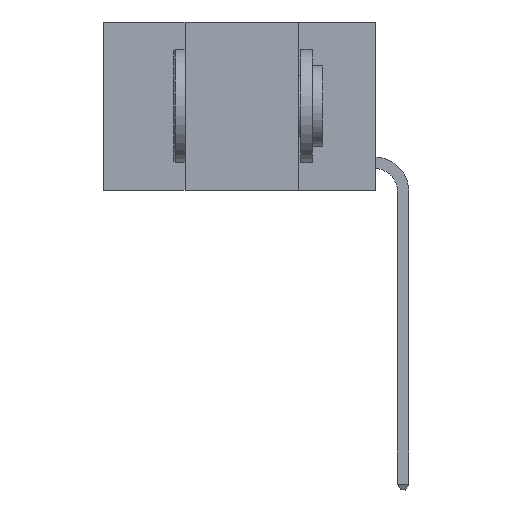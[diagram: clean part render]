
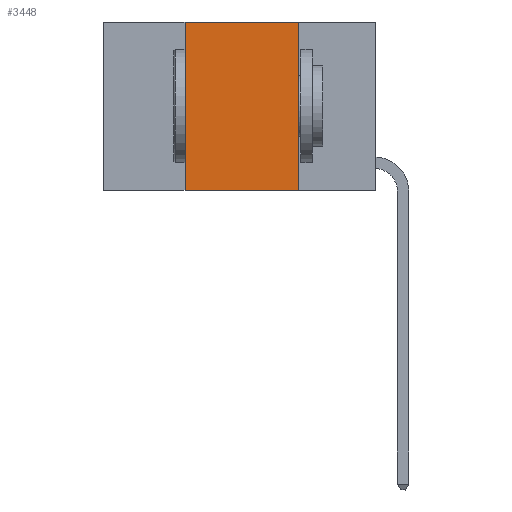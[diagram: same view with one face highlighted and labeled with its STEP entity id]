
A CAD part, left-side view. The second image highlights one B-rep face of the part: STEP entity #3448.
In plain terms, the highlighted planar face has unit normal (-1, 0, 0).
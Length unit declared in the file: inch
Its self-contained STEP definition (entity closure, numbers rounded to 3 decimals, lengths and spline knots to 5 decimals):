
#687 = EDGE_CURVE ( 'NONE', #4513, #5849, #4733, .T. ) ;
#817 = VECTOR ( 'NONE', #2018, 39.37008 ) ;
#1158 = VECTOR ( 'NONE', #10260, 39.37008 ) ;
#2018 = DIRECTION ( 'NONE',  ( 0., -1., 0. ) ) ;
#2038 = VERTEX_POINT ( 'NONE', #10872 ) ;
#2383 = ORIENTED_EDGE ( 'NONE', *, *, #13498, .F. ) ;
#2482 = ORIENTED_EDGE ( 'NONE', *, *, #4453, .F. ) ;
#3216 = PLANE ( 'NONE',  #8801 ) ;
#3448 = ADVANCED_FACE ( 'NONE', ( #8709 ), #3216, .F. ) ;
#3645 = ORIENTED_EDGE ( 'NONE', *, *, #687, .F. ) ;
#3662 = ORIENTED_EDGE ( 'NONE', *, *, #15948, .T. ) ;
#4453 = EDGE_CURVE ( 'NONE', #5849, #2038, #7474, .T. ) ;
#4513 = VERTEX_POINT ( 'NONE', #4835 ) ;
#4561 = DIRECTION ( 'NONE',  ( 1., 0., 0. ) ) ;
#4733 = LINE ( 'NONE', #6243, #1158 ) ;
#4770 = DIRECTION ( 'NONE',  ( 0., -1., 0. ) ) ;
#4835 = CARTESIAN_POINT ( 'NONE',  ( 0., 0.42, -0.37 ) ) ;
#4949 = VECTOR ( 'NONE', #4770, 39.37008 ) ;
#5364 = LINE ( 'NONE', #11214, #4949 ) ;
#5849 = VERTEX_POINT ( 'NONE', #7764 ) ;
#6049 = DIRECTION ( 'NONE',  ( 0., 0., -1. ) ) ;
#6243 = CARTESIAN_POINT ( 'NONE',  ( 0., 0.42, 0. ) ) ;
#6273 = LINE ( 'NONE', #11174, #12700 ) ;
#7474 = LINE ( 'NONE', #14957, #817 ) ;
#7544 = CARTESIAN_POINT ( 'NONE',  ( 0., 0.17, -0.37 ) ) ;
#7764 = CARTESIAN_POINT ( 'NONE',  ( 0., 0.42, 0. ) ) ;
#8709 = FACE_OUTER_BOUND ( 'NONE', #13694, .T. ) ;
#8801 = AXIS2_PLACEMENT_3D ( 'NONE', #12283, #4561, #13556 ) ;
#9128 = VERTEX_POINT ( 'NONE', #7544 ) ;
#10260 = DIRECTION ( 'NONE',  ( 0., 0., 1. ) ) ;
#10872 = CARTESIAN_POINT ( 'NONE',  ( 0., 0.17, 0. ) ) ;
#11174 = CARTESIAN_POINT ( 'NONE',  ( 0., 0.17, 0. ) ) ;
#11214 = CARTESIAN_POINT ( 'NONE',  ( 0., 0.6, -0.37 ) ) ;
#12283 = CARTESIAN_POINT ( 'NONE',  ( 0., 0.6, 0. ) ) ;
#12700 = VECTOR ( 'NONE', #6049, 39.37008 ) ;
#13498 = EDGE_CURVE ( 'NONE', #2038, #9128, #6273, .T. ) ;
#13556 = DIRECTION ( 'NONE',  ( 0., 0., -1. ) ) ;
#13694 = EDGE_LOOP ( 'NONE', ( #2383, #2482, #3645, #3662 ) ) ;
#14957 = CARTESIAN_POINT ( 'NONE',  ( 0., 0.6, 0. ) ) ;
#15948 = EDGE_CURVE ( 'NONE', #4513, #9128, #5364, .T. ) ;
